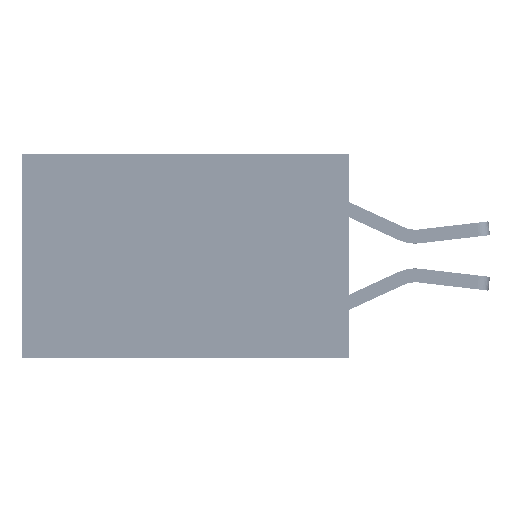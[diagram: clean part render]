
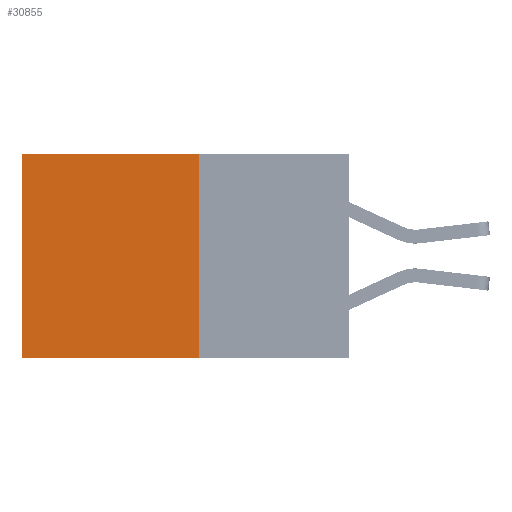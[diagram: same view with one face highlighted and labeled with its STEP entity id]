
A CAD part, left-side view. The second image highlights one B-rep face of the part: STEP entity #30855.
In plain terms, the highlighted planar face has unit normal (-1, 0, 0).
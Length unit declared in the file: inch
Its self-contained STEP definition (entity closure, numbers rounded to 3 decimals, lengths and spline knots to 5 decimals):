
#658 = DIRECTION ( 'NONE',  ( 0., 0., -1. ) ) ;
#781 = FACE_OUTER_BOUND ( 'NONE', #1460, .T. ) ;
#787 = DIRECTION ( 'NONE',  ( 0., 1., 0. ) ) ;
#1460 = EDGE_LOOP ( 'NONE', ( #14216, #34692, #32945, #12582 ) ) ;
#7963 = VERTEX_POINT ( 'NONE', #14775 ) ;
#9091 = DIRECTION ( 'NONE',  ( 0., 1., 0. ) ) ;
#10218 = LINE ( 'NONE', #32196, #17764 ) ;
#12582 = ORIENTED_EDGE ( 'NONE', *, *, #30872, .T. ) ;
#13310 = CARTESIAN_POINT ( 'NONE',  ( 0.277, 0.27, -0.37 ) ) ;
#13829 = EDGE_CURVE ( 'NONE', #25884, #7963, #28657, .T. ) ;
#14216 = ORIENTED_EDGE ( 'NONE', *, *, #30473, .T. ) ;
#14747 = CARTESIAN_POINT ( 'NONE',  ( 0.277, 0.27, -0.37 ) ) ;
#14775 = CARTESIAN_POINT ( 'NONE',  ( 0.277, 0.59, -0.37 ) ) ;
#17697 = DIRECTION ( 'NONE',  ( 1., 0., 0. ) ) ;
#17764 = VECTOR ( 'NONE', #35009, 39.37008 ) ;
#18294 = VERTEX_POINT ( 'NONE', #28918 ) ;
#20856 = AXIS2_PLACEMENT_3D ( 'NONE', #14747, #17697, #658 ) ;
#21757 = LINE ( 'NONE', #24226, #35785 ) ;
#23473 = CARTESIAN_POINT ( 'NONE',  ( 0.277, 0.27, 0. ) ) ;
#24045 = VECTOR ( 'NONE', #787, 39.37008 ) ;
#24226 = CARTESIAN_POINT ( 'NONE',  ( 0.277, 0.59, -0.37 ) ) ;
#25884 = VERTEX_POINT ( 'NONE', #13310 ) ;
#28657 = LINE ( 'NONE', #31721, #29515 ) ;
#28918 = CARTESIAN_POINT ( 'NONE',  ( 0.277, 0.27, 0. ) ) ;
#29230 = EDGE_CURVE ( 'NONE', #18294, #25884, #10218, .T. ) ;
#29515 = VECTOR ( 'NONE', #9091, 39.37008 ) ;
#30473 = EDGE_CURVE ( 'NONE', #33111, #7963, #21757, .T. ) ;
#30855 = ADVANCED_FACE ( 'NONE', ( #781 ), #34591, .F. ) ;
#30872 = EDGE_CURVE ( 'NONE', #18294, #33111, #31474, .T. ) ;
#31474 = LINE ( 'NONE', #23473, #24045 ) ;
#31721 = CARTESIAN_POINT ( 'NONE',  ( 0.277, 0.27, -0.37 ) ) ;
#32196 = CARTESIAN_POINT ( 'NONE',  ( 0.277, 0.27, -0.37 ) ) ;
#32945 = ORIENTED_EDGE ( 'NONE', *, *, #29230, .F. ) ;
#33111 = VERTEX_POINT ( 'NONE', #34581 ) ;
#34581 = CARTESIAN_POINT ( 'NONE',  ( 0.277, 0.59, 0. ) ) ;
#34591 = PLANE ( 'NONE',  #20856 ) ;
#34692 = ORIENTED_EDGE ( 'NONE', *, *, #13829, .F. ) ;
#35009 = DIRECTION ( 'NONE',  ( 0., 0., -1. ) ) ;
#35454 = DIRECTION ( 'NONE',  ( 0., 0., -1. ) ) ;
#35785 = VECTOR ( 'NONE', #35454, 39.37008 ) ;
